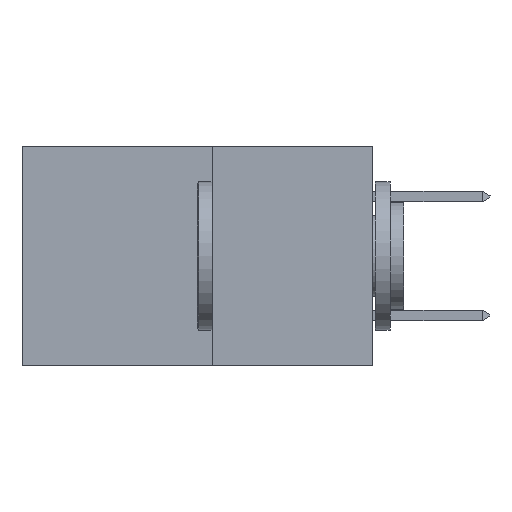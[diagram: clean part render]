
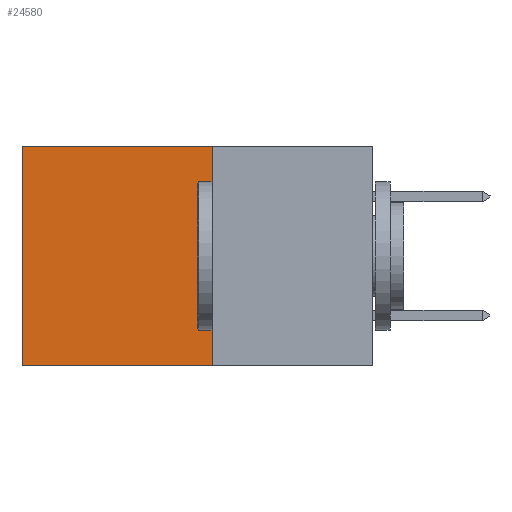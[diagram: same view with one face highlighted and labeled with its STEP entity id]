
A CAD part, left-side view. The second image highlights one B-rep face of the part: STEP entity #24580.
In plain terms, the highlighted planar face has unit normal (-1, 0, 0).
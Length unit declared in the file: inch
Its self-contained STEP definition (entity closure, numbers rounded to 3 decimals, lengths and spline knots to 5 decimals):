
#517 = EDGE_CURVE ( 'NONE', #26940, #30790, #32759, .T. ) ;
#1657 = AXIS2_PLACEMENT_3D ( 'NONE', #29534, #13580, #32178 ) ;
#2252 = EDGE_CURVE ( 'NONE', #26940, #12935, #12730, .T. ) ;
#3380 = EDGE_CURVE ( 'NONE', #30790, #27181, #34223, .T. ) ;
#5536 = CARTESIAN_POINT ( 'NONE',  ( 0.277, 0.27, 0. ) ) ;
#6682 = LINE ( 'NONE', #21428, #20879 ) ;
#9774 = DIRECTION ( 'NONE',  ( 0., 0., -1. ) ) ;
#12730 = LINE ( 'NONE', #28509, #19002 ) ;
#12935 = VERTEX_POINT ( 'NONE', #27601 ) ;
#13580 = DIRECTION ( 'NONE',  ( 1., 0., 0. ) ) ;
#14611 = DIRECTION ( 'NONE',  ( 0., 1., 0. ) ) ;
#14860 = ORIENTED_EDGE ( 'NONE', *, *, #517, .T. ) ;
#16647 = CARTESIAN_POINT ( 'NONE',  ( 0.277, 0.27, 0. ) ) ;
#17439 = ORIENTED_EDGE ( 'NONE', *, *, #2252, .F. ) ;
#19002 = VECTOR ( 'NONE', #9774, 39.37008 ) ;
#20155 = FACE_OUTER_BOUND ( 'NONE', #25611, .T. ) ;
#20879 = VECTOR ( 'NONE', #24093, 39.37008 ) ;
#21428 = CARTESIAN_POINT ( 'NONE',  ( 0.277, 0.27, -0.37 ) ) ;
#21544 = PLANE ( 'NONE',  #1657 ) ;
#24093 = DIRECTION ( 'NONE',  ( 0., 1., 0. ) ) ;
#24580 = ADVANCED_FACE ( 'NONE', ( #20155 ), #21544, .F. ) ;
#24827 = DIRECTION ( 'NONE',  ( 0., 0., -1. ) ) ;
#25611 = EDGE_LOOP ( 'NONE', ( #27311, #27061, #17439, #14860 ) ) ;
#26593 = CARTESIAN_POINT ( 'NONE',  ( 0.277, 0.59, -0.37 ) ) ;
#26940 = VERTEX_POINT ( 'NONE', #16647 ) ;
#27061 = ORIENTED_EDGE ( 'NONE', *, *, #33974, .F. ) ;
#27181 = VERTEX_POINT ( 'NONE', #33295 ) ;
#27311 = ORIENTED_EDGE ( 'NONE', *, *, #3380, .T. ) ;
#27601 = CARTESIAN_POINT ( 'NONE',  ( 0.277, 0.27, -0.37 ) ) ;
#27725 = CARTESIAN_POINT ( 'NONE',  ( 0.277, 0.59, 0. ) ) ;
#28509 = CARTESIAN_POINT ( 'NONE',  ( 0.277, 0.27, -0.37 ) ) ;
#29534 = CARTESIAN_POINT ( 'NONE',  ( 0.277, 0.27, -0.37 ) ) ;
#30790 = VERTEX_POINT ( 'NONE', #27725 ) ;
#31937 = VECTOR ( 'NONE', #14611, 39.37008 ) ;
#32178 = DIRECTION ( 'NONE',  ( 0., 0., -1. ) ) ;
#32759 = LINE ( 'NONE', #5536, #31937 ) ;
#33295 = CARTESIAN_POINT ( 'NONE',  ( 0.277, 0.59, -0.37 ) ) ;
#33406 = VECTOR ( 'NONE', #24827, 39.37008 ) ;
#33974 = EDGE_CURVE ( 'NONE', #12935, #27181, #6682, .T. ) ;
#34223 = LINE ( 'NONE', #26593, #33406 ) ;
